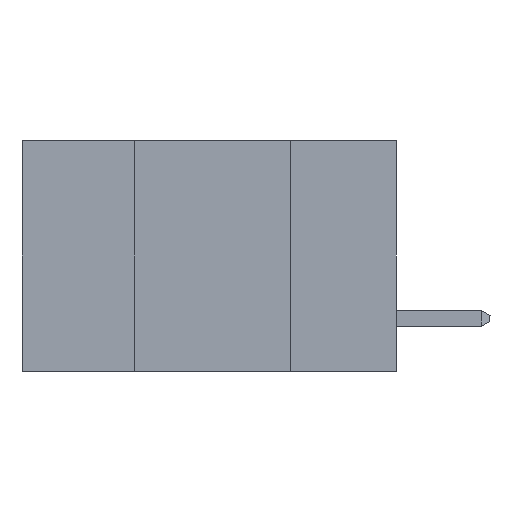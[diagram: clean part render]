
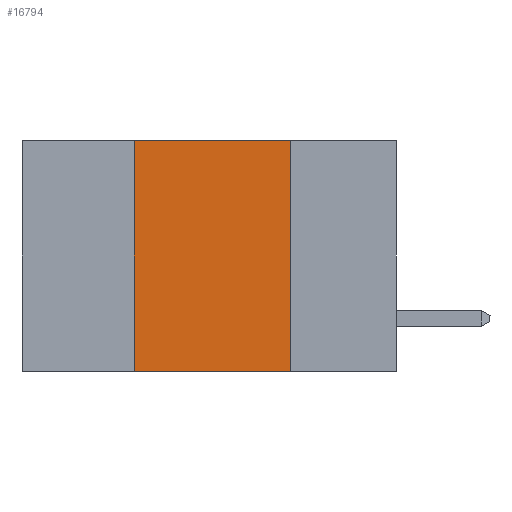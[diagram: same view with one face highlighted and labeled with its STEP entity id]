
A CAD part, left-side view. The second image highlights one B-rep face of the part: STEP entity #16794.
In plain terms, the highlighted planar face has unit normal (-1, 0, 0).
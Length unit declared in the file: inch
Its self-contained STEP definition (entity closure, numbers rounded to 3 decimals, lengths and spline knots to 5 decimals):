
#1008 = EDGE_LOOP ( 'NONE', ( #17694, #21111, #12456, #5990 ) ) ;
#2404 = DIRECTION ( 'NONE',  ( 1., 0., 0. ) ) ;
#3303 = EDGE_CURVE ( 'NONE', #6282, #4781, #3855, .T. ) ;
#3855 = LINE ( 'NONE', #18306, #17765 ) ;
#3906 = EDGE_CURVE ( 'NONE', #4781, #19018, #5180, .T. ) ;
#4618 = VECTOR ( 'NONE', #18235, 39.37008 ) ;
#4781 = VERTEX_POINT ( 'NONE', #5986 ) ;
#5180 = LINE ( 'NONE', #18278, #4618 ) ;
#5908 = VECTOR ( 'NONE', #11348, 39.37008 ) ;
#5986 = CARTESIAN_POINT ( 'NONE',  ( 0., 0.17, 0. ) ) ;
#5990 = ORIENTED_EDGE ( 'NONE', *, *, #13116, .T. ) ;
#6282 = VERTEX_POINT ( 'NONE', #18319 ) ;
#7240 = VERTEX_POINT ( 'NONE', #19465 ) ;
#7489 = CARTESIAN_POINT ( 'NONE',  ( 0., 0.17, -0.37 ) ) ;
#7646 = PLANE ( 'NONE',  #17533 ) ;
#8415 = DIRECTION ( 'NONE',  ( 0., -1., 0. ) ) ;
#8422 = CARTESIAN_POINT ( 'NONE',  ( 0., 0.6, -0.37 ) ) ;
#9382 = VECTOR ( 'NONE', #8415, 39.37008 ) ;
#11348 = DIRECTION ( 'NONE',  ( 0., 0., 1. ) ) ;
#12140 = FACE_OUTER_BOUND ( 'NONE', #1008, .T. ) ;
#12456 = ORIENTED_EDGE ( 'NONE', *, *, #16172, .F. ) ;
#12913 = CARTESIAN_POINT ( 'NONE',  ( 0., 0.6, 0. ) ) ;
#13116 = EDGE_CURVE ( 'NONE', #7240, #19018, #18060, .T. ) ;
#14625 = DIRECTION ( 'NONE',  ( 0., 0., -1. ) ) ;
#15740 = LINE ( 'NONE', #16484, #5908 ) ;
#16172 = EDGE_CURVE ( 'NONE', #7240, #6282, #15740, .T. ) ;
#16484 = CARTESIAN_POINT ( 'NONE',  ( 0., 0.42, -0.37 ) ) ;
#16794 = ADVANCED_FACE ( 'NONE', ( #12140 ), #7646, .F. ) ;
#17533 = AXIS2_PLACEMENT_3D ( 'NONE', #12913, #2404, #14625 ) ;
#17694 = ORIENTED_EDGE ( 'NONE', *, *, #3906, .F. ) ;
#17765 = VECTOR ( 'NONE', #18260, 39.37008 ) ;
#18060 = LINE ( 'NONE', #8422, #9382 ) ;
#18235 = DIRECTION ( 'NONE',  ( 0., 0., -1. ) ) ;
#18260 = DIRECTION ( 'NONE',  ( 0., -1., 0. ) ) ;
#18278 = CARTESIAN_POINT ( 'NONE',  ( 0., 0.17, -0.37 ) ) ;
#18306 = CARTESIAN_POINT ( 'NONE',  ( 0., 0.6, 0. ) ) ;
#18319 = CARTESIAN_POINT ( 'NONE',  ( 0., 0.42, 0. ) ) ;
#19018 = VERTEX_POINT ( 'NONE', #7489 ) ;
#19465 = CARTESIAN_POINT ( 'NONE',  ( 0., 0.42, -0.37 ) ) ;
#21111 = ORIENTED_EDGE ( 'NONE', *, *, #3303, .F. ) ;
